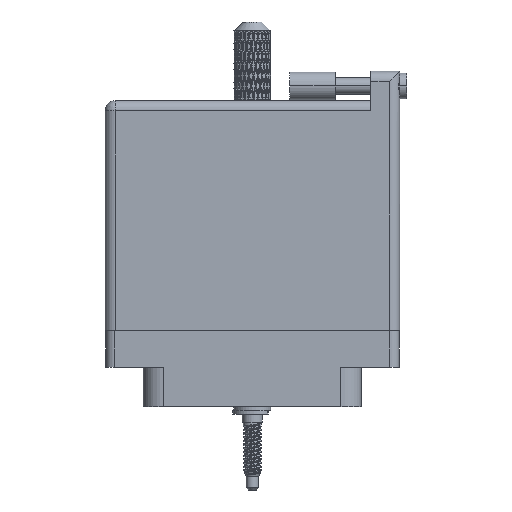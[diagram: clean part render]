
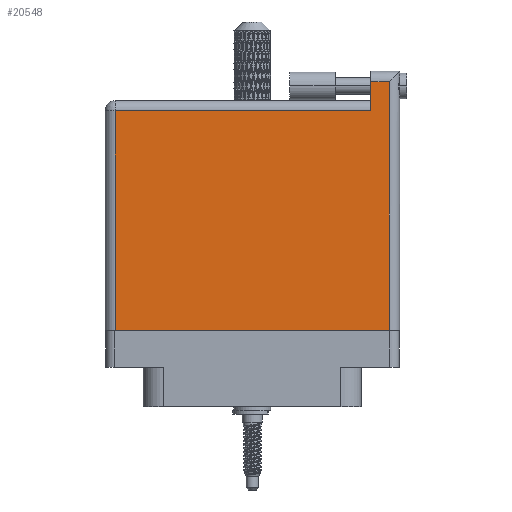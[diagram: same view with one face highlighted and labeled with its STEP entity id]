
A CAD part, front view. The second image highlights one B-rep face of the part: STEP entity #20548.
In plain terms, the highlighted face is planar.
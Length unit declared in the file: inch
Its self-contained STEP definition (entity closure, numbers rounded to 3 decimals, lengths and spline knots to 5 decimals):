
#1261 = CARTESIAN_POINT ( 'NONE',  ( -0.934, -0.1, 0.4495 ) ) ;
#3156 = CARTESIAN_POINT ( 'NONE',  ( -1.004, -0.1, 0.4495 ) ) ;
#4946 = VECTOR ( 'NONE', #100079, 39.37008 ) ;
#6038 = EDGE_CURVE ( 'NONE', #88451, #47222, #36953, .T. ) ;
#6595 = VECTOR ( 'NONE', #35276, 39.37008 ) ;
#7027 = VECTOR ( 'NONE', #66243, 39.37008 ) ;
#9006 = DIRECTION ( 'NONE',  ( 0., -1., 0. ) ) ;
#15403 = CARTESIAN_POINT ( 'NONE',  ( 0.934, 1.666, 0.4495 ) ) ;
#20548 = ADVANCED_FACE ( 'NONE', ( #37932 ), #80180, .F. ) ;
#21239 = EDGE_CURVE ( 'NONE', #100989, #37746, #104067, .T. ) ;
#22663 = EDGE_CURVE ( 'NONE', #47222, #100989, #40162, .T. ) ;
#24535 = ORIENTED_EDGE ( 'NONE', *, *, #67835, .T. ) ;
#26738 = CARTESIAN_POINT ( 'NONE',  ( -1.004, 1.396, 0.4495 ) ) ;
#27240 = VECTOR ( 'NONE', #89427, 39.37008 ) ;
#31812 = CARTESIAN_POINT ( 'NONE',  ( -1.004, 1.466, 0.4495 ) ) ;
#32162 = DIRECTION ( 'NONE',  ( -1., 0., 0. ) ) ;
#35276 = DIRECTION ( 'NONE',  ( 1., 0., 0. ) ) ;
#36303 = CARTESIAN_POINT ( 'NONE',  ( 0.807, 1.596, 0.4495 ) ) ;
#36953 = LINE ( 'NONE', #58866, #4946 ) ;
#37746 = VERTEX_POINT ( 'NONE', #1261 ) ;
#37932 = FACE_OUTER_BOUND ( 'NONE', #53603, .T. ) ;
#40008 = ORIENTED_EDGE ( 'NONE', *, *, #22663, .T. ) ;
#40162 = LINE ( 'NONE', #26738, #7027 ) ;
#42345 = LINE ( 'NONE', #3156, #6595 ) ;
#47222 = VERTEX_POINT ( 'NONE', #74218 ) ;
#51551 = EDGE_CURVE ( 'NONE', #105436, #90601, #76842, .T. ) ;
#51970 = ORIENTED_EDGE ( 'NONE', *, *, #6038, .T. ) ;
#52287 = AXIS2_PLACEMENT_3D ( 'NONE', #31812, #56379, #32162 ) ;
#53603 = EDGE_LOOP ( 'NONE', ( #24535, #77621, #90246, #51970, #40008, #97826 ) ) ;
#56379 = DIRECTION ( 'NONE',  ( 0., 0., -1. ) ) ;
#58866 = CARTESIAN_POINT ( 'NONE',  ( 0.807, 1.666, 0.4495 ) ) ;
#62521 = CARTESIAN_POINT ( 'NONE',  ( -1.004, 1.596, 0.4495 ) ) ;
#65748 = LINE ( 'NONE', #62521, #91275 ) ;
#66243 = DIRECTION ( 'NONE',  ( -1., 0., 0. ) ) ;
#67835 = EDGE_CURVE ( 'NONE', #37746, #105436, #42345, .T. ) ;
#69679 = CARTESIAN_POINT ( 'NONE',  ( 0.934, -0.1, 0.4495 ) ) ;
#74218 = CARTESIAN_POINT ( 'NONE',  ( 0.807, 1.396, 0.4495 ) ) ;
#74572 = CARTESIAN_POINT ( 'NONE',  ( -0.934, -0.1, 0.4495 ) ) ;
#76842 = LINE ( 'NONE', #15403, #27240 ) ;
#77621 = ORIENTED_EDGE ( 'NONE', *, *, #51551, .T. ) ;
#80180 = PLANE ( 'NONE',  #52287 ) ;
#80430 = EDGE_CURVE ( 'NONE', #90601, #88451, #65748, .T. ) ;
#82851 = CARTESIAN_POINT ( 'NONE',  ( -0.934, 1.396, 0.4495 ) ) ;
#84846 = CARTESIAN_POINT ( 'NONE',  ( 0.934, 1.596, 0.4495 ) ) ;
#87495 = VECTOR ( 'NONE', #9006, 39.37008 ) ;
#88451 = VERTEX_POINT ( 'NONE', #36303 ) ;
#89427 = DIRECTION ( 'NONE',  ( 0., 1., 0. ) ) ;
#90246 = ORIENTED_EDGE ( 'NONE', *, *, #80430, .T. ) ;
#90601 = VERTEX_POINT ( 'NONE', #84846 ) ;
#91275 = VECTOR ( 'NONE', #102365, 39.37008 ) ;
#97826 = ORIENTED_EDGE ( 'NONE', *, *, #21239, .T. ) ;
#100079 = DIRECTION ( 'NONE',  ( 0., -1., 0. ) ) ;
#100989 = VERTEX_POINT ( 'NONE', #82851 ) ;
#102365 = DIRECTION ( 'NONE',  ( -1., 0., 0. ) ) ;
#104067 = LINE ( 'NONE', #74572, #87495 ) ;
#105436 = VERTEX_POINT ( 'NONE', #69679 ) ;
